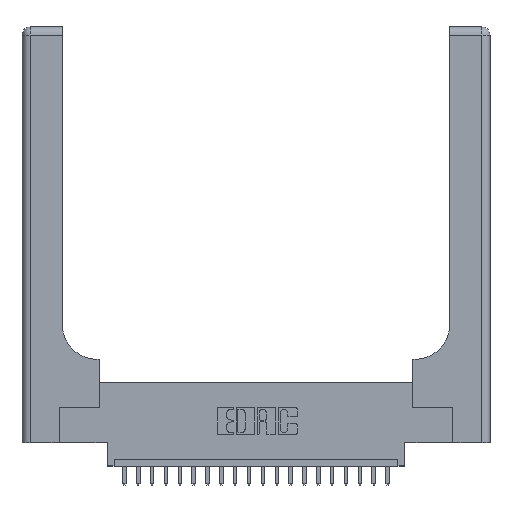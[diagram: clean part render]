
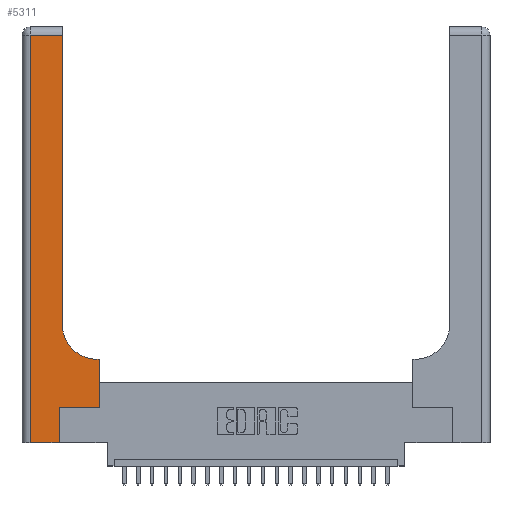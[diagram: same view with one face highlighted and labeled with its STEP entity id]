
A CAD part, top view. The second image highlights one B-rep face of the part: STEP entity #5311.
In plain terms, the highlighted planar face has unit normal (0, 0, 1).
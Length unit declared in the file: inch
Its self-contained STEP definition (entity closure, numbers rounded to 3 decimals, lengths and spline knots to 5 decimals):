
#270 = VECTOR ( 'NONE', #11816, 39.37008 ) ;
#298 = CARTESIAN_POINT ( 'NONE',  ( 0., 3., 0.37 ) ) ;
#721 = DIRECTION ( 'NONE',  ( 1., 0., 0. ) ) ;
#769 = DIRECTION ( 'NONE',  ( -1., 0., 0. ) ) ;
#1029 = CARTESIAN_POINT ( 'NONE',  ( 0.2915, 0.85, 0.37 ) ) ;
#1366 = CARTESIAN_POINT ( 'NONE',  ( 0.5415, 0.6, 0.37 ) ) ;
#1369 = CARTESIAN_POINT ( 'NONE',  ( 0.5585, 0.25, 0.37 ) ) ;
#1423 = CARTESIAN_POINT ( 'NONE',  ( 0.06, 0., 0.37 ) ) ;
#1436 = CARTESIAN_POINT ( 'NONE',  ( 0.269, 0., 0.37 ) ) ;
#2036 = CARTESIAN_POINT ( 'NONE',  ( 0.2915, 2.94, 0.37 ) ) ;
#2422 = CARTESIAN_POINT ( 'NONE',  ( 0., 2.94, 0.37 ) ) ;
#2488 = CARTESIAN_POINT ( 'NONE',  ( 0.2915, 0.6, 0.37 ) ) ;
#3097 = ORIENTED_EDGE ( 'NONE', *, *, #12005, .T. ) ;
#3309 = CIRCLE ( 'NONE', #11333, 0.25 ) ;
#3318 = VECTOR ( 'NONE', #769, 39.37008 ) ;
#3344 = ORIENTED_EDGE ( 'NONE', *, *, #22450, .T. ) ;
#3578 = VECTOR ( 'NONE', #17764, 39.37008 ) ;
#4197 = CARTESIAN_POINT ( 'NONE',  ( 0.5415, 0.85, 0.37 ) ) ;
#4669 = VERTEX_POINT ( 'NONE', #1369 ) ;
#4851 = VERTEX_POINT ( 'NONE', #20290 ) ;
#5103 = LINE ( 'NONE', #20762, #270 ) ;
#5311 = ADVANCED_FACE ( 'NONE', ( #10492 ), #12812, .F. ) ;
#5422 = EDGE_CURVE ( 'NONE', #6050, #8570, #5103, .T. ) ;
#5563 = EDGE_LOOP ( 'NONE', ( #22665, #3097, #13269, #12570, #5679, #3344, #21157, #16786, #7541 ) ) ;
#5679 = ORIENTED_EDGE ( 'NONE', *, *, #7282, .T. ) ;
#5866 = EDGE_CURVE ( 'NONE', #11890, #4851, #12721, .T. ) ;
#6050 = VERTEX_POINT ( 'NONE', #1029 ) ;
#6107 = VERTEX_POINT ( 'NONE', #11214 ) ;
#6239 = LINE ( 'NONE', #2422, #22019 ) ;
#6429 = CARTESIAN_POINT ( 'NONE',  ( 0.269, 0.25, 0.37 ) ) ;
#6949 = VECTOR ( 'NONE', #22444, 39.37008 ) ;
#7266 = EDGE_CURVE ( 'NONE', #8629, #11890, #17958, .T. ) ;
#7282 = EDGE_CURVE ( 'NONE', #4851, #6107, #16552, .T. ) ;
#7541 = ORIENTED_EDGE ( 'NONE', *, *, #7568, .T. ) ;
#7568 = EDGE_CURVE ( 'NONE', #12807, #6050, #3309, .T. ) ;
#7719 = DIRECTION ( 'NONE',  ( 0., 0., -1. ) ) ;
#8570 = VERTEX_POINT ( 'NONE', #2036 ) ;
#8629 = VERTEX_POINT ( 'NONE', #9882 ) ;
#9768 = VECTOR ( 'NONE', #721, 39.37008 ) ;
#9882 = CARTESIAN_POINT ( 'NONE',  ( 0.06, 2.94, 0.37 ) ) ;
#10492 = FACE_OUTER_BOUND ( 'NONE', #5563, .T. ) ;
#10904 = DIRECTION ( 'NONE',  ( 0., 0., -1. ) ) ;
#11063 = DIRECTION ( 'NONE',  ( -1., 0., 0. ) ) ;
#11214 = CARTESIAN_POINT ( 'NONE',  ( 0.269, 0.25, 0.37 ) ) ;
#11333 = AXIS2_PLACEMENT_3D ( 'NONE', #4197, #7719, #20358 ) ;
#11726 = LINE ( 'NONE', #20633, #6949 ) ;
#11816 = DIRECTION ( 'NONE',  ( 0., 1., 0. ) ) ;
#11871 = VECTOR ( 'NONE', #17308, 39.37008 ) ;
#11890 = VERTEX_POINT ( 'NONE', #1423 ) ;
#12005 = EDGE_CURVE ( 'NONE', #8570, #8629, #6239, .T. ) ;
#12391 = CARTESIAN_POINT ( 'NONE',  ( 0.06, 3., 0.37 ) ) ;
#12467 = LINE ( 'NONE', #6429, #9768 ) ;
#12570 = ORIENTED_EDGE ( 'NONE', *, *, #5866, .T. ) ;
#12721 = LINE ( 'NONE', #22620, #11871 ) ;
#12807 = VERTEX_POINT ( 'NONE', #1366 ) ;
#12812 = PLANE ( 'NONE',  #16705 ) ;
#13216 = VECTOR ( 'NONE', #21419, 39.37008 ) ;
#13269 = ORIENTED_EDGE ( 'NONE', *, *, #7266, .T. ) ;
#13570 = EDGE_CURVE ( 'NONE', #16548, #12807, #15456, .T. ) ;
#15456 = LINE ( 'NONE', #2488, #3318 ) ;
#16548 = VERTEX_POINT ( 'NONE', #20480 ) ;
#16552 = LINE ( 'NONE', #1436, #3578 ) ;
#16705 = AXIS2_PLACEMENT_3D ( 'NONE', #298, #10904, #11063 ) ;
#16786 = ORIENTED_EDGE ( 'NONE', *, *, #13570, .T. ) ;
#17308 = DIRECTION ( 'NONE',  ( 1., 0., 0. ) ) ;
#17764 = DIRECTION ( 'NONE',  ( 0., 1., 0. ) ) ;
#17958 = LINE ( 'NONE', #12391, #13216 ) ;
#19162 = EDGE_CURVE ( 'NONE', #4669, #16548, #11726, .T. ) ;
#20290 = CARTESIAN_POINT ( 'NONE',  ( 0.269, 0., 0.37 ) ) ;
#20358 = DIRECTION ( 'NONE',  ( 1., 0., 0. ) ) ;
#20480 = CARTESIAN_POINT ( 'NONE',  ( 0.5585, 0.6, 0.37 ) ) ;
#20633 = CARTESIAN_POINT ( 'NONE',  ( 0.5585, 0.25, 0.37 ) ) ;
#20762 = CARTESIAN_POINT ( 'NONE',  ( 0.2915, 3., 0.37 ) ) ;
#21157 = ORIENTED_EDGE ( 'NONE', *, *, #19162, .T. ) ;
#21419 = DIRECTION ( 'NONE',  ( 0., -1., 0. ) ) ;
#21945 = DIRECTION ( 'NONE',  ( -1., 0., 0. ) ) ;
#22019 = VECTOR ( 'NONE', #21945, 39.37008 ) ;
#22444 = DIRECTION ( 'NONE',  ( 0., 1., 0. ) ) ;
#22450 = EDGE_CURVE ( 'NONE', #6107, #4669, #12467, .T. ) ;
#22620 = CARTESIAN_POINT ( 'NONE',  ( 0., 0., 0.37 ) ) ;
#22665 = ORIENTED_EDGE ( 'NONE', *, *, #5422, .T. ) ;
